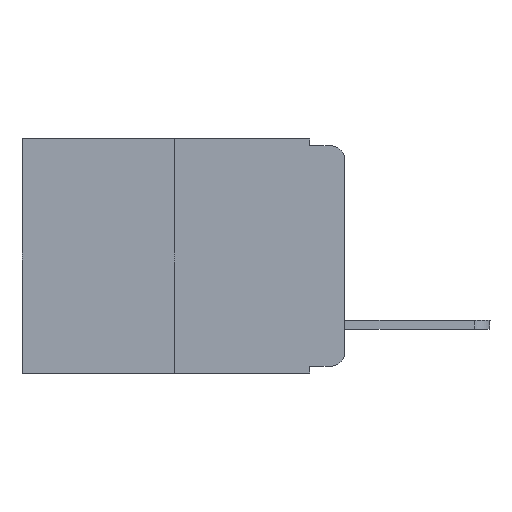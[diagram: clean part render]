
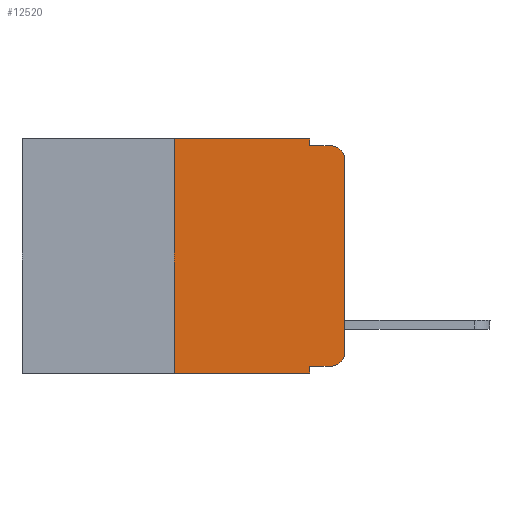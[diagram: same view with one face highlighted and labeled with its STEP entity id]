
A CAD part, left-side view. The second image highlights one B-rep face of the part: STEP entity #12520.
In plain terms, the highlighted planar face has unit normal (-1, 0, 0).
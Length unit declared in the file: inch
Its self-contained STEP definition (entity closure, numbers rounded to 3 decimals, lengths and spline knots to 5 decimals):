
#62 = DIRECTION ( 'NONE',  ( 0., 0., 1. ) ) ;
#192 = DIRECTION ( 'NONE',  ( 1., 0., 0. ) ) ;
#333 = CARTESIAN_POINT ( 'NONE',  ( 0., 0., -0.313 ) ) ;
#337 = DIRECTION ( 'NONE',  ( 0., 0., -1. ) ) ;
#451 = LINE ( 'NONE', #10070, #3784 ) ;
#487 = VECTOR ( 'NONE', #15443, 39.37008 ) ;
#624 = EDGE_LOOP ( 'NONE', ( #18306, #13837, #15126, #22314, #21131, #20444, #8809, #17573, #2923, #3519 ) ) ;
#787 = VERTEX_POINT ( 'NONE', #9558 ) ;
#1133 = VERTEX_POINT ( 'NONE', #3487 ) ;
#1318 = LINE ( 'NONE', #6294, #12892 ) ;
#1985 = FACE_OUTER_BOUND ( 'NONE', #624, .T. ) ;
#2002 = EDGE_CURVE ( 'NONE', #16938, #8528, #14476, .T. ) ;
#2359 = AXIS2_PLACEMENT_3D ( 'NONE', #16660, #11319, #20113 ) ;
#2586 = CARTESIAN_POINT ( 'NONE',  ( 0., 0.051, -0.01 ) ) ;
#2923 = ORIENTED_EDGE ( 'NONE', *, *, #18386, .T. ) ;
#2928 = EDGE_CURVE ( 'NONE', #787, #4702, #6159, .T. ) ;
#3086 = VECTOR ( 'NONE', #62, 39.37008 ) ;
#3409 = CARTESIAN_POINT ( 'NONE',  ( 0., 0.051, -0.01 ) ) ;
#3487 = CARTESIAN_POINT ( 'NONE',  ( 0., 0.051, 0. ) ) ;
#3519 = ORIENTED_EDGE ( 'NONE', *, *, #2928, .T. ) ;
#3676 = CARTESIAN_POINT ( 'NONE',  ( 0., 0.02, -0.03 ) ) ;
#3784 = VECTOR ( 'NONE', #4246, 39.37008 ) ;
#4246 = DIRECTION ( 'NONE',  ( 0., -1., 0. ) ) ;
#4393 = EDGE_CURVE ( 'NONE', #16880, #18118, #1318, .T. ) ;
#4702 = VERTEX_POINT ( 'NONE', #333 ) ;
#4803 = CARTESIAN_POINT ( 'NONE',  ( 0., 0.25, -0.343 ) ) ;
#5037 = VERTEX_POINT ( 'NONE', #3409 ) ;
#5450 = CARTESIAN_POINT ( 'NONE',  ( 0., 0.473, 0. ) ) ;
#5915 = AXIS2_PLACEMENT_3D ( 'NONE', #3676, #18380, #337 ) ;
#6159 = CIRCLE ( 'NONE', #2359, 0.02 ) ;
#6294 = CARTESIAN_POINT ( 'NONE',  ( 0., 0.051, 0. ) ) ;
#6385 = EDGE_CURVE ( 'NONE', #16938, #18118, #17830, .T. ) ;
#7382 = VERTEX_POINT ( 'NONE', #21664 ) ;
#7806 = CIRCLE ( 'NONE', #5915, 0.02 ) ;
#7885 = EDGE_CURVE ( 'NONE', #7382, #15751, #7806, .T. ) ;
#8528 = VERTEX_POINT ( 'NONE', #12412 ) ;
#8607 = CARTESIAN_POINT ( 'NONE',  ( 0., 0.051, -0.333 ) ) ;
#8809 = ORIENTED_EDGE ( 'NONE', *, *, #6385, .T. ) ;
#9437 = CARTESIAN_POINT ( 'NONE',  ( 0., 0.051, -0.343 ) ) ;
#9490 = LINE ( 'NONE', #11750, #487 ) ;
#9558 = CARTESIAN_POINT ( 'NONE',  ( 0., 0.02, -0.333 ) ) ;
#9786 = CARTESIAN_POINT ( 'NONE',  ( 0., 0.051, -0.333 ) ) ;
#10070 = CARTESIAN_POINT ( 'NONE',  ( 0., 0.473, 0. ) ) ;
#10682 = CARTESIAN_POINT ( 'NONE',  ( 0., 0.473, -0.343 ) ) ;
#10856 = EDGE_CURVE ( 'NONE', #8528, #1133, #451, .T. ) ;
#11066 = CARTESIAN_POINT ( 'NONE',  ( 0., 0.02, -0.01 ) ) ;
#11319 = DIRECTION ( 'NONE',  ( -1., 0., 0. ) ) ;
#11750 = CARTESIAN_POINT ( 'NONE',  ( 0., 0.051, 0. ) ) ;
#11821 = LINE ( 'NONE', #20628, #14012 ) ;
#11905 = DIRECTION ( 'NONE',  ( 0., 0., -1. ) ) ;
#12282 = EDGE_CURVE ( 'NONE', #5037, #15751, #18892, .T. ) ;
#12412 = CARTESIAN_POINT ( 'NONE',  ( 0., 0.25, 0. ) ) ;
#12520 = ADVANCED_FACE ( 'NONE', ( #1985 ), #12585, .F. ) ;
#12585 = PLANE ( 'NONE',  #22105 ) ;
#12892 = VECTOR ( 'NONE', #11905, 39.37008 ) ;
#13412 = EDGE_CURVE ( 'NONE', #1133, #5037, #9490, .T. ) ;
#13731 = DIRECTION ( 'NONE',  ( 0., 0., 1. ) ) ;
#13837 = ORIENTED_EDGE ( 'NONE', *, *, #7885, .T. ) ;
#14012 = VECTOR ( 'NONE', #13731, 39.37008 ) ;
#14476 = LINE ( 'NONE', #16257, #3086 ) ;
#15126 = ORIENTED_EDGE ( 'NONE', *, *, #12282, .F. ) ;
#15443 = DIRECTION ( 'NONE',  ( 0., 0., -1. ) ) ;
#15751 = VERTEX_POINT ( 'NONE', #11066 ) ;
#16257 = CARTESIAN_POINT ( 'NONE',  ( 0., 0.25, 0. ) ) ;
#16660 = CARTESIAN_POINT ( 'NONE',  ( 0., 0.02, -0.313 ) ) ;
#16843 = EDGE_CURVE ( 'NONE', #4702, #7382, #11821, .T. ) ;
#16880 = VERTEX_POINT ( 'NONE', #9786 ) ;
#16938 = VERTEX_POINT ( 'NONE', #4803 ) ;
#17573 = ORIENTED_EDGE ( 'NONE', *, *, #4393, .F. ) ;
#17830 = LINE ( 'NONE', #10682, #19154 ) ;
#18118 = VERTEX_POINT ( 'NONE', #9437 ) ;
#18306 = ORIENTED_EDGE ( 'NONE', *, *, #16843, .T. ) ;
#18380 = DIRECTION ( 'NONE',  ( -1., 0., 0. ) ) ;
#18386 = EDGE_CURVE ( 'NONE', #16880, #787, #21565, .T. ) ;
#18892 = LINE ( 'NONE', #2586, #20946 ) ;
#19154 = VECTOR ( 'NONE', #23384, 39.37008 ) ;
#20113 = DIRECTION ( 'NONE',  ( 0., 0., -1. ) ) ;
#20444 = ORIENTED_EDGE ( 'NONE', *, *, #2002, .F. ) ;
#20628 = CARTESIAN_POINT ( 'NONE',  ( 0., 0., 0. ) ) ;
#20895 = VECTOR ( 'NONE', #21335, 39.37008 ) ;
#20946 = VECTOR ( 'NONE', #22567, 39.37008 ) ;
#21131 = ORIENTED_EDGE ( 'NONE', *, *, #10856, .F. ) ;
#21335 = DIRECTION ( 'NONE',  ( 0., -1., 0. ) ) ;
#21565 = LINE ( 'NONE', #8607, #20895 ) ;
#21664 = CARTESIAN_POINT ( 'NONE',  ( 0., 0., -0.03 ) ) ;
#22079 = DIRECTION ( 'NONE',  ( 0., 0., -1. ) ) ;
#22105 = AXIS2_PLACEMENT_3D ( 'NONE', #5450, #192, #22079 ) ;
#22314 = ORIENTED_EDGE ( 'NONE', *, *, #13412, .F. ) ;
#22567 = DIRECTION ( 'NONE',  ( 0., -1., 0. ) ) ;
#23384 = DIRECTION ( 'NONE',  ( 0., -1., 0. ) ) ;
